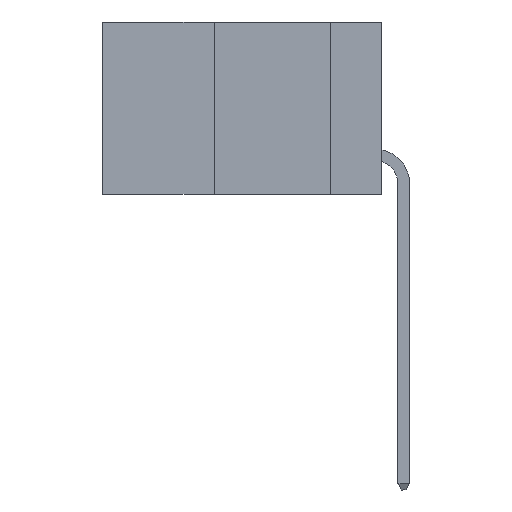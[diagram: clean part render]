
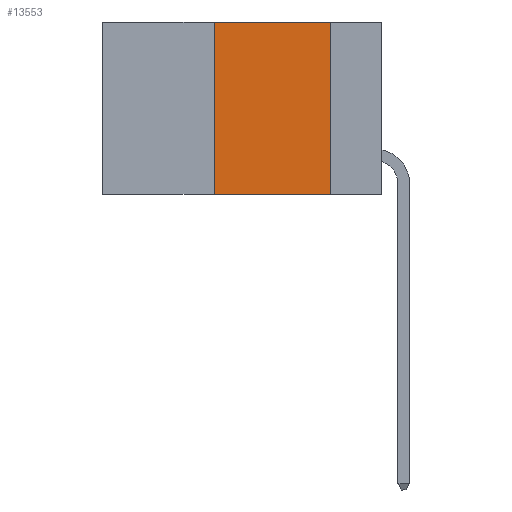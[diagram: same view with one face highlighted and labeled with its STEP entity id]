
A CAD part, left-side view. The second image highlights one B-rep face of the part: STEP entity #13553.
In plain terms, the highlighted planar face has unit normal (-1, 0, 0).
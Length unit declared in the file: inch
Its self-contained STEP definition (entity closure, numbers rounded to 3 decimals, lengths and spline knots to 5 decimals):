
#329 = CARTESIAN_POINT ( 'NONE',  ( 0., 0.11, -0.37 ) ) ;
#986 = LINE ( 'NONE', #10682, #8901 ) ;
#1633 = CARTESIAN_POINT ( 'NONE',  ( 0., 0.6, 0. ) ) ;
#2324 = FACE_OUTER_BOUND ( 'NONE', #9804, .T. ) ;
#2734 = DIRECTION ( 'NONE',  ( 0., 0., 1. ) ) ;
#3409 = LINE ( 'NONE', #1633, #6615 ) ;
#3504 = CARTESIAN_POINT ( 'NONE',  ( 0., 0.11, 0. ) ) ;
#4020 = EDGE_CURVE ( 'NONE', #5617, #7370, #986, .T. ) ;
#4046 = VECTOR ( 'NONE', #19808, 39.37008 ) ;
#4547 = AXIS2_PLACEMENT_3D ( 'NONE', #15265, #6040, #16774 ) ;
#5617 = VERTEX_POINT ( 'NONE', #3504 ) ;
#5837 = ORIENTED_EDGE ( 'NONE', *, *, #11124, .F. ) ;
#6040 = DIRECTION ( 'NONE',  ( 1., 0., 0. ) ) ;
#6339 = ORIENTED_EDGE ( 'NONE', *, *, #14092, .T. ) ;
#6615 = VECTOR ( 'NONE', #11080, 39.37008 ) ;
#7370 = VERTEX_POINT ( 'NONE', #329 ) ;
#7994 = DIRECTION ( 'NONE',  ( 0., 0., -1. ) ) ;
#8214 = LINE ( 'NONE', #16762, #4046 ) ;
#8901 = VECTOR ( 'NONE', #7994, 39.37008 ) ;
#9746 = CARTESIAN_POINT ( 'NONE',  ( 0., 0.36, 0. ) ) ;
#9804 = EDGE_LOOP ( 'NONE', ( #17594, #5837, #10012, #6339 ) ) ;
#10012 = ORIENTED_EDGE ( 'NONE', *, *, #12861, .F. ) ;
#10263 = CARTESIAN_POINT ( 'NONE',  ( 0., 0.36, -0.37 ) ) ;
#10682 = CARTESIAN_POINT ( 'NONE',  ( 0., 0.11, 0. ) ) ;
#10780 = VERTEX_POINT ( 'NONE', #10263 ) ;
#11080 = DIRECTION ( 'NONE',  ( 0., -1., 0. ) ) ;
#11124 = EDGE_CURVE ( 'NONE', #19191, #5617, #3409, .T. ) ;
#12121 = CARTESIAN_POINT ( 'NONE',  ( 0., 0.36, 0. ) ) ;
#12238 = PLANE ( 'NONE',  #4547 ) ;
#12861 = EDGE_CURVE ( 'NONE', #10780, #19191, #15957, .T. ) ;
#13553 = ADVANCED_FACE ( 'NONE', ( #2324 ), #12238, .F. ) ;
#14092 = EDGE_CURVE ( 'NONE', #10780, #7370, #8214, .T. ) ;
#15265 = CARTESIAN_POINT ( 'NONE',  ( 0., 0.6, 0. ) ) ;
#15957 = LINE ( 'NONE', #12121, #19482 ) ;
#16762 = CARTESIAN_POINT ( 'NONE',  ( 0., 0.6, -0.37 ) ) ;
#16774 = DIRECTION ( 'NONE',  ( 0., 0., -1. ) ) ;
#17594 = ORIENTED_EDGE ( 'NONE', *, *, #4020, .F. ) ;
#19191 = VERTEX_POINT ( 'NONE', #9746 ) ;
#19482 = VECTOR ( 'NONE', #2734, 39.37008 ) ;
#19808 = DIRECTION ( 'NONE',  ( 0., -1., 0. ) ) ;
